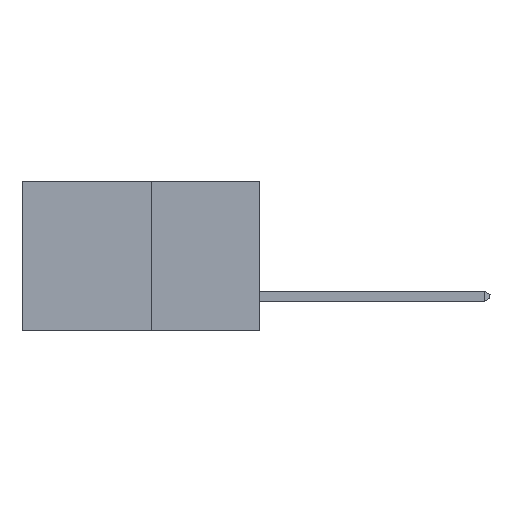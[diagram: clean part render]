
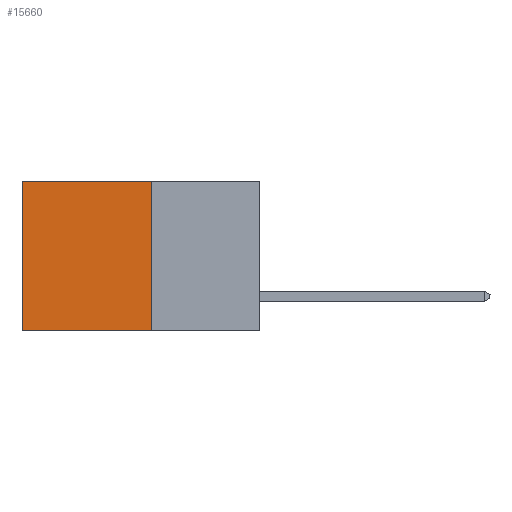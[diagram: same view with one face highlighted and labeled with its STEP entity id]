
A CAD part, left-side view. The second image highlights one B-rep face of the part: STEP entity #15660.
In plain terms, the highlighted planar face has unit normal (-1, 0, 0).
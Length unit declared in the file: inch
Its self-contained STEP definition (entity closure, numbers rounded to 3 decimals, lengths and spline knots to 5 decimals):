
#50 = ORIENTED_EDGE ( 'NONE', *, *, #2693, .F. ) ;
#200 = ORIENTED_EDGE ( 'NONE', *, *, #381, .F. ) ;
#381 = EDGE_CURVE ( 'NONE', #16146, #14784, #1683, .T. ) ;
#386 = ORIENTED_EDGE ( 'NONE', *, *, #15480, .T. ) ;
#619 = EDGE_CURVE ( 'NONE', #10414, #5479, #5184, .T. ) ;
#1683 = LINE ( 'NONE', #10778, #9625 ) ;
#1948 = VECTOR ( 'NONE', #6647, 39.37008 ) ;
#2693 = EDGE_CURVE ( 'NONE', #14784, #5479, #17106, .T. ) ;
#2915 = DIRECTION ( 'NONE',  ( 0., 0., -1. ) ) ;
#3036 = FACE_OUTER_BOUND ( 'NONE', #12120, .T. ) ;
#3352 = DIRECTION ( 'NONE',  ( 0., 0., -1. ) ) ;
#5153 = CARTESIAN_POINT ( 'NONE',  ( 0.277, 0.27, 0. ) ) ;
#5184 = LINE ( 'NONE', #13672, #15938 ) ;
#5479 = VERTEX_POINT ( 'NONE', #15872 ) ;
#5608 = DIRECTION ( 'NONE',  ( 1., 0., 0. ) ) ;
#6647 = DIRECTION ( 'NONE',  ( 0., 1., 0. ) ) ;
#8259 = CARTESIAN_POINT ( 'NONE',  ( 0.277, 0.27, -0.37 ) ) ;
#8886 = DIRECTION ( 'NONE',  ( 0., 1., 0. ) ) ;
#9460 = LINE ( 'NONE', #13671, #1948 ) ;
#9625 = VECTOR ( 'NONE', #3352, 39.37008 ) ;
#10414 = VERTEX_POINT ( 'NONE', #11972 ) ;
#10778 = CARTESIAN_POINT ( 'NONE',  ( 0.277, 0.27, -0.37 ) ) ;
#11215 = PLANE ( 'NONE',  #12580 ) ;
#11972 = CARTESIAN_POINT ( 'NONE',  ( 0.277, 0.59, 0. ) ) ;
#12120 = EDGE_LOOP ( 'NONE', ( #15192, #50, #200, #386 ) ) ;
#12580 = AXIS2_PLACEMENT_3D ( 'NONE', #14041, #5608, #15446 ) ;
#13671 = CARTESIAN_POINT ( 'NONE',  ( 0.277, 0.27, 0. ) ) ;
#13672 = CARTESIAN_POINT ( 'NONE',  ( 0.277, 0.59, -0.37 ) ) ;
#14041 = CARTESIAN_POINT ( 'NONE',  ( 0.277, 0.27, -0.37 ) ) ;
#14784 = VERTEX_POINT ( 'NONE', #14910 ) ;
#14910 = CARTESIAN_POINT ( 'NONE',  ( 0.277, 0.27, -0.37 ) ) ;
#15192 = ORIENTED_EDGE ( 'NONE', *, *, #619, .T. ) ;
#15446 = DIRECTION ( 'NONE',  ( 0., 0., -1. ) ) ;
#15480 = EDGE_CURVE ( 'NONE', #16146, #10414, #9460, .T. ) ;
#15660 = ADVANCED_FACE ( 'NONE', ( #3036 ), #11215, .F. ) ;
#15872 = CARTESIAN_POINT ( 'NONE',  ( 0.277, 0.59, -0.37 ) ) ;
#15938 = VECTOR ( 'NONE', #2915, 39.37008 ) ;
#16146 = VERTEX_POINT ( 'NONE', #5153 ) ;
#16265 = VECTOR ( 'NONE', #8886, 39.37008 ) ;
#17106 = LINE ( 'NONE', #8259, #16265 ) ;
